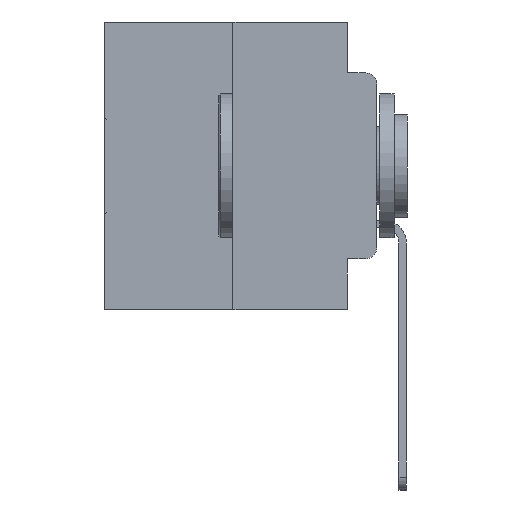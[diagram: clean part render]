
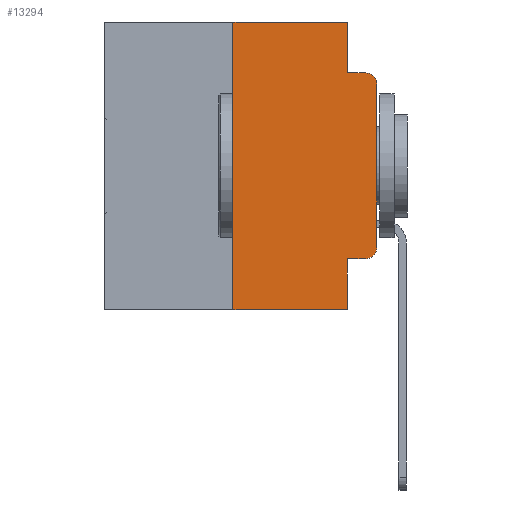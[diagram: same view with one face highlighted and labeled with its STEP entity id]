
A CAD part, left-side view. The second image highlights one B-rep face of the part: STEP entity #13294.
In plain terms, the highlighted planar face has unit normal (-1, 0, 0).
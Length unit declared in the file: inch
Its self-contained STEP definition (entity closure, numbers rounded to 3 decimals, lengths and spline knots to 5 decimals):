
#236 = CARTESIAN_POINT ( 'NONE',  ( 0., 0.051, -0.4115 ) ) ;
#764 = DIRECTION ( 'NONE',  ( 0., 0., 1. ) ) ;
#862 = VECTOR ( 'NONE', #18898, 39.37008 ) ;
#874 = EDGE_CURVE ( 'NONE', #9572, #21574, #6215, .T. ) ;
#1759 = AXIS2_PLACEMENT_3D ( 'NONE', #10977, #27926, #13365 ) ;
#2211 = CARTESIAN_POINT ( 'NONE',  ( 0., 0.051, 0. ) ) ;
#2560 = VECTOR ( 'NONE', #764, 39.37008 ) ;
#2619 = CARTESIAN_POINT ( 'NONE',  ( 0., 0.473, 0. ) ) ;
#2663 = CARTESIAN_POINT ( 'NONE',  ( 0., 0., 0. ) ) ;
#2801 = FACE_OUTER_BOUND ( 'NONE', #18210, .T. ) ;
#3832 = CARTESIAN_POINT ( 'NONE',  ( 0., 0.473, -0.5 ) ) ;
#3956 = CARTESIAN_POINT ( 'NONE',  ( 0., 0.25, -0.5 ) ) ;
#4036 = VECTOR ( 'NONE', #29904, 39.37008 ) ;
#4649 = CARTESIAN_POINT ( 'NONE',  ( 0., 0.051, -0.4115 ) ) ;
#5285 = VECTOR ( 'NONE', #29247, 39.37008 ) ;
#6183 = EDGE_CURVE ( 'NONE', #18202, #9572, #15615, .T. ) ;
#6215 = CIRCLE ( 'NONE', #21889, 0.02 ) ;
#6805 = EDGE_CURVE ( 'NONE', #26164, #18202, #30438, .T. ) ;
#7137 = DIRECTION ( 'NONE',  ( 0., -1., 0. ) ) ;
#7791 = ORIENTED_EDGE ( 'NONE', *, *, #6805, .T. ) ;
#8011 = ORIENTED_EDGE ( 'NONE', *, *, #29657, .F. ) ;
#8316 = CARTESIAN_POINT ( 'NONE',  ( 0., 0.02, -0.4115 ) ) ;
#8609 = CARTESIAN_POINT ( 'NONE',  ( 0., 0.25, 0. ) ) ;
#8648 = VECTOR ( 'NONE', #11279, 39.37008 ) ;
#8769 = ORIENTED_EDGE ( 'NONE', *, *, #26407, .F. ) ;
#9572 = VERTEX_POINT ( 'NONE', #23971 ) ;
#9656 = VERTEX_POINT ( 'NONE', #4649 ) ;
#10153 = EDGE_CURVE ( 'NONE', #9656, #26164, #17143, .T. ) ;
#10977 = CARTESIAN_POINT ( 'NONE',  ( 0., 0.02, -0.3915 ) ) ;
#11279 = DIRECTION ( 'NONE',  ( 0., -1., 0. ) ) ;
#11322 = VERTEX_POINT ( 'NONE', #13050 ) ;
#12556 = VECTOR ( 'NONE', #7137, 39.37008 ) ;
#12879 = AXIS2_PLACEMENT_3D ( 'NONE', #16744, #31456, #16858 ) ;
#13050 = CARTESIAN_POINT ( 'NONE',  ( 0., 0.051, 0. ) ) ;
#13294 = ADVANCED_FACE ( 'NONE', ( #2801 ), #29025, .F. ) ;
#13355 = EDGE_CURVE ( 'NONE', #9656, #16657, #19089, .T. ) ;
#13365 = DIRECTION ( 'NONE',  ( 0., 0., -1. ) ) ;
#13881 = CARTESIAN_POINT ( 'NONE',  ( 0., 0.051, -0.0885 ) ) ;
#14208 = ORIENTED_EDGE ( 'NONE', *, *, #13355, .F. ) ;
#14239 = LINE ( 'NONE', #28677, #862 ) ;
#14644 = EDGE_CURVE ( 'NONE', #26368, #11322, #25508, .T. ) ;
#14881 = LINE ( 'NONE', #3832, #27084 ) ;
#15615 = LINE ( 'NONE', #2663, #22898 ) ;
#16657 = VERTEX_POINT ( 'NONE', #19347 ) ;
#16744 = CARTESIAN_POINT ( 'NONE',  ( 0., 0.473, 0. ) ) ;
#16858 = DIRECTION ( 'NONE',  ( 0., 0., -1. ) ) ;
#17143 = LINE ( 'NONE', #236, #4036 ) ;
#17495 = DIRECTION ( 'NONE',  ( 0., 0., 1. ) ) ;
#18202 = VERTEX_POINT ( 'NONE', #25031 ) ;
#18210 = EDGE_LOOP ( 'NONE', ( #21266, #21324, #8011, #8769, #27776, #26685, #31636, #14208, #26818, #7791 ) ) ;
#18898 = DIRECTION ( 'NONE',  ( 0., 0., -1. ) ) ;
#19089 = LINE ( 'NONE', #2211, #5285 ) ;
#19347 = CARTESIAN_POINT ( 'NONE',  ( 0., 0.051, -0.5 ) ) ;
#20552 = VERTEX_POINT ( 'NONE', #3956 ) ;
#21266 = ORIENTED_EDGE ( 'NONE', *, *, #6183, .T. ) ;
#21324 = ORIENTED_EDGE ( 'NONE', *, *, #874, .T. ) ;
#21511 = LINE ( 'NONE', #8609, #2560 ) ;
#21519 = EDGE_CURVE ( 'NONE', #20552, #26368, #21511, .T. ) ;
#21574 = VERTEX_POINT ( 'NONE', #23391 ) ;
#21633 = VERTEX_POINT ( 'NONE', #13881 ) ;
#21889 = AXIS2_PLACEMENT_3D ( 'NONE', #29699, #29628, #29246 ) ;
#22898 = VECTOR ( 'NONE', #17495, 39.37008 ) ;
#23372 = CARTESIAN_POINT ( 'NONE',  ( 0., 0.051, -0.0885 ) ) ;
#23391 = CARTESIAN_POINT ( 'NONE',  ( 0., 0.02, -0.0885 ) ) ;
#23971 = CARTESIAN_POINT ( 'NONE',  ( 0., 0., -0.1085 ) ) ;
#24425 = EDGE_CURVE ( 'NONE', #20552, #16657, #14881, .T. ) ;
#25031 = CARTESIAN_POINT ( 'NONE',  ( 0., 0., -0.3915 ) ) ;
#25508 = LINE ( 'NONE', #2619, #12556 ) ;
#25957 = DIRECTION ( 'NONE',  ( 0., -1., 0. ) ) ;
#26050 = CARTESIAN_POINT ( 'NONE',  ( 0., 0.25, 0. ) ) ;
#26164 = VERTEX_POINT ( 'NONE', #8316 ) ;
#26368 = VERTEX_POINT ( 'NONE', #26050 ) ;
#26407 = EDGE_CURVE ( 'NONE', #11322, #21633, #14239, .T. ) ;
#26685 = ORIENTED_EDGE ( 'NONE', *, *, #21519, .F. ) ;
#26818 = ORIENTED_EDGE ( 'NONE', *, *, #10153, .T. ) ;
#27084 = VECTOR ( 'NONE', #25957, 39.37008 ) ;
#27776 = ORIENTED_EDGE ( 'NONE', *, *, #14644, .F. ) ;
#27926 = DIRECTION ( 'NONE',  ( -1., 0., 0. ) ) ;
#28026 = LINE ( 'NONE', #23372, #8648 ) ;
#28677 = CARTESIAN_POINT ( 'NONE',  ( 0., 0.051, 0. ) ) ;
#29025 = PLANE ( 'NONE',  #12879 ) ;
#29246 = DIRECTION ( 'NONE',  ( 0., 0., -1. ) ) ;
#29247 = DIRECTION ( 'NONE',  ( 0., 0., -1. ) ) ;
#29628 = DIRECTION ( 'NONE',  ( -1., 0., 0. ) ) ;
#29657 = EDGE_CURVE ( 'NONE', #21633, #21574, #28026, .T. ) ;
#29699 = CARTESIAN_POINT ( 'NONE',  ( 0., 0.02, -0.1085 ) ) ;
#29904 = DIRECTION ( 'NONE',  ( 0., -1., 0. ) ) ;
#30438 = CIRCLE ( 'NONE', #1759, 0.02 ) ;
#31456 = DIRECTION ( 'NONE',  ( 1., 0., 0. ) ) ;
#31636 = ORIENTED_EDGE ( 'NONE', *, *, #24425, .T. ) ;
